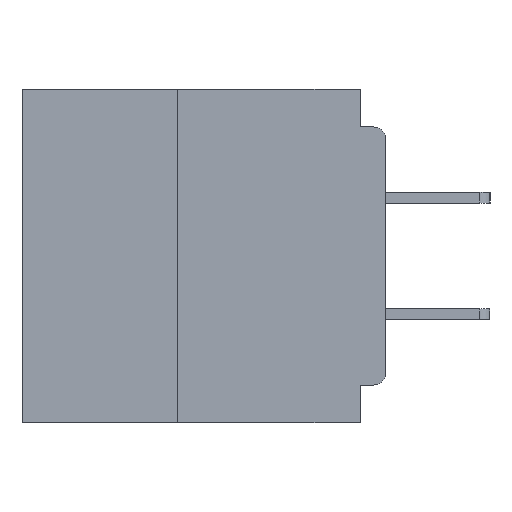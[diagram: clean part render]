
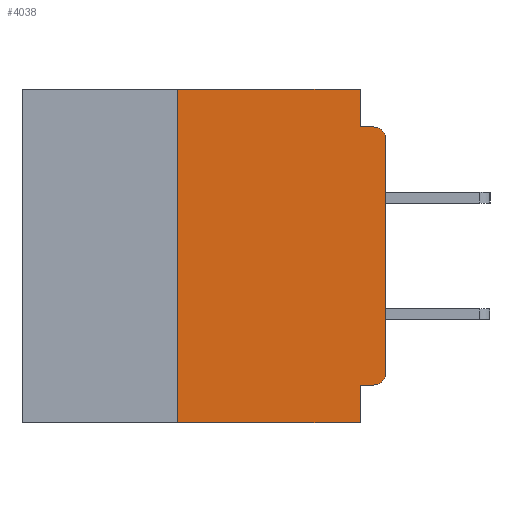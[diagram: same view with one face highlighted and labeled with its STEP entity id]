
A CAD part, left-side view. The second image highlights one B-rep face of the part: STEP entity #4038.
In plain terms, the highlighted planar face has unit normal (-1, 0, 0).
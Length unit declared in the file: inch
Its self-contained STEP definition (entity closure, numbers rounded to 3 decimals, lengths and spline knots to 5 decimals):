
#603 = DIRECTION ( 'NONE',  ( 0., 0., -1. ) ) ;
#946 = VECTOR ( 'NONE', #4618, 39.37008 ) ;
#1047 = ORIENTED_EDGE ( 'NONE', *, *, #15902, .T. ) ;
#1572 = CARTESIAN_POINT ( 'NONE',  ( 0., 0.031, 0. ) ) ;
#1636 = CARTESIAN_POINT ( 'NONE',  ( 0., 0., -0.355 ) ) ;
#2380 = CARTESIAN_POINT ( 'NONE',  ( 0., 0.031, -0.045 ) ) ;
#3191 = EDGE_CURVE ( 'NONE', #14133, #14926, #33543, .T. ) ;
#3691 = VERTEX_POINT ( 'NONE', #11919 ) ;
#4038 = ADVANCED_FACE ( 'NONE', ( #18070 ), #27724, .F. ) ;
#4454 = ORIENTED_EDGE ( 'NONE', *, *, #3191, .F. ) ;
#4618 = DIRECTION ( 'NONE',  ( 0., 0., -1. ) ) ;
#5223 = DIRECTION ( 'NONE',  ( 0., 1., 0. ) ) ;
#5489 = VECTOR ( 'NONE', #40925, 39.37008 ) ;
#5492 = VECTOR ( 'NONE', #19135, 39.37008 ) ;
#6193 = CARTESIAN_POINT ( 'NONE',  ( 0., 0.25, 0. ) ) ;
#6438 = EDGE_CURVE ( 'NONE', #9483, #26176, #23150, .T. ) ;
#6444 = CARTESIAN_POINT ( 'NONE',  ( 0., 0.015, -0.355 ) ) ;
#6653 = EDGE_CURVE ( 'NONE', #9483, #31273, #24288, .T. ) ;
#6787 = VECTOR ( 'NONE', #603, 39.37008 ) ;
#7107 = CIRCLE ( 'NONE', #43862, 0.015 ) ;
#7591 = VECTOR ( 'NONE', #12393, 39.37008 ) ;
#8892 = ORIENTED_EDGE ( 'NONE', *, *, #32130, .F. ) ;
#9258 = LINE ( 'NONE', #25743, #946 ) ;
#9483 = VERTEX_POINT ( 'NONE', #44171 ) ;
#10170 = DIRECTION ( 'NONE',  ( 1., 0., 0. ) ) ;
#10602 = ORIENTED_EDGE ( 'NONE', *, *, #29965, .F. ) ;
#10964 = AXIS2_PLACEMENT_3D ( 'NONE', #34128, #13068, #37622 ) ;
#11337 = VECTOR ( 'NONE', #24433, 39.37008 ) ;
#11665 = EDGE_CURVE ( 'NONE', #39422, #18505, #28375, .T. ) ;
#11753 = DIRECTION ( 'NONE',  ( -1., 0., 0. ) ) ;
#11919 = CARTESIAN_POINT ( 'NONE',  ( 0., 0.031, -0.355 ) ) ;
#12393 = DIRECTION ( 'NONE',  ( 0., 0., 1. ) ) ;
#13068 = DIRECTION ( 'NONE',  ( -1., 0., 0. ) ) ;
#14133 = VERTEX_POINT ( 'NONE', #2380 ) ;
#14206 = CARTESIAN_POINT ( 'NONE',  ( 0., 0., -0.34 ) ) ;
#14926 = VERTEX_POINT ( 'NONE', #40661 ) ;
#15604 = CARTESIAN_POINT ( 'NONE',  ( 0., 0.437, -0.4 ) ) ;
#15902 = EDGE_CURVE ( 'NONE', #19029, #14926, #7107, .T. ) ;
#16236 = ORIENTED_EDGE ( 'NONE', *, *, #11665, .T. ) ;
#18070 = FACE_OUTER_BOUND ( 'NONE', #32858, .T. ) ;
#18505 = VERTEX_POINT ( 'NONE', #14206 ) ;
#19029 = VERTEX_POINT ( 'NONE', #31232 ) ;
#19135 = DIRECTION ( 'NONE',  ( 0., -1., 0. ) ) ;
#19564 = ORIENTED_EDGE ( 'NONE', *, *, #6653, .F. ) ;
#23150 = LINE ( 'NONE', #15604, #5492 ) ;
#23502 = CARTESIAN_POINT ( 'NONE',  ( 0., 0., -0.045 ) ) ;
#24042 = CARTESIAN_POINT ( 'NONE',  ( 0., 0.437, 0. ) ) ;
#24288 = LINE ( 'NONE', #44846, #41792 ) ;
#24433 = DIRECTION ( 'NONE',  ( 0., -1., 0. ) ) ;
#25743 = CARTESIAN_POINT ( 'NONE',  ( 0., 0.031, 0. ) ) ;
#25761 = EDGE_CURVE ( 'NONE', #43222, #14133, #9258, .T. ) ;
#25885 = LINE ( 'NONE', #1636, #32996 ) ;
#25990 = EDGE_CURVE ( 'NONE', #18505, #19029, #28521, .T. ) ;
#26046 = EDGE_CURVE ( 'NONE', #3691, #26176, #43494, .T. ) ;
#26176 = VERTEX_POINT ( 'NONE', #41348 ) ;
#27426 = DIRECTION ( 'NONE',  ( 0., 0., 1. ) ) ;
#27724 = PLANE ( 'NONE',  #36923 ) ;
#28375 = CIRCLE ( 'NONE', #10964, 0.015 ) ;
#28521 = LINE ( 'NONE', #40457, #7591 ) ;
#28962 = LINE ( 'NONE', #45358, #11337 ) ;
#29965 = EDGE_CURVE ( 'NONE', #39422, #3691, #25885, .T. ) ;
#31232 = CARTESIAN_POINT ( 'NONE',  ( 0., 0., -0.06 ) ) ;
#31273 = VERTEX_POINT ( 'NONE', #6193 ) ;
#32130 = EDGE_CURVE ( 'NONE', #31273, #43222, #28962, .T. ) ;
#32376 = CARTESIAN_POINT ( 'NONE',  ( 0., 0.031, -0.4 ) ) ;
#32816 = CARTESIAN_POINT ( 'NONE',  ( 0., 0.015, -0.06 ) ) ;
#32858 = EDGE_LOOP ( 'NONE', ( #45035, #1047, #4454, #44317, #8892, #19564, #37371, #42548, #10602, #16236 ) ) ;
#32996 = VECTOR ( 'NONE', #5223, 39.37008 ) ;
#33543 = LINE ( 'NONE', #23502, #5489 ) ;
#34128 = CARTESIAN_POINT ( 'NONE',  ( 0., 0.015, -0.34 ) ) ;
#34754 = DIRECTION ( 'NONE',  ( 0., 0., -1. ) ) ;
#36303 = DIRECTION ( 'NONE',  ( 0., 0., -1. ) ) ;
#36923 = AXIS2_PLACEMENT_3D ( 'NONE', #24042, #10170, #34754 ) ;
#37371 = ORIENTED_EDGE ( 'NONE', *, *, #6438, .T. ) ;
#37622 = DIRECTION ( 'NONE',  ( 0., 0., -1. ) ) ;
#39422 = VERTEX_POINT ( 'NONE', #6444 ) ;
#40457 = CARTESIAN_POINT ( 'NONE',  ( 0., 0., 0. ) ) ;
#40661 = CARTESIAN_POINT ( 'NONE',  ( 0., 0.015, -0.045 ) ) ;
#40925 = DIRECTION ( 'NONE',  ( 0., -1., 0. ) ) ;
#41348 = CARTESIAN_POINT ( 'NONE',  ( 0., 0.031, -0.4 ) ) ;
#41792 = VECTOR ( 'NONE', #27426, 39.37008 ) ;
#42548 = ORIENTED_EDGE ( 'NONE', *, *, #26046, .F. ) ;
#43222 = VERTEX_POINT ( 'NONE', #1572 ) ;
#43494 = LINE ( 'NONE', #32376, #6787 ) ;
#43862 = AXIS2_PLACEMENT_3D ( 'NONE', #32816, #11753, #36303 ) ;
#44171 = CARTESIAN_POINT ( 'NONE',  ( 0., 0.25, -0.4 ) ) ;
#44317 = ORIENTED_EDGE ( 'NONE', *, *, #25761, .F. ) ;
#44846 = CARTESIAN_POINT ( 'NONE',  ( 0., 0.25, -0.4 ) ) ;
#45035 = ORIENTED_EDGE ( 'NONE', *, *, #25990, .T. ) ;
#45358 = CARTESIAN_POINT ( 'NONE',  ( 0., 0.437, 0. ) ) ;
